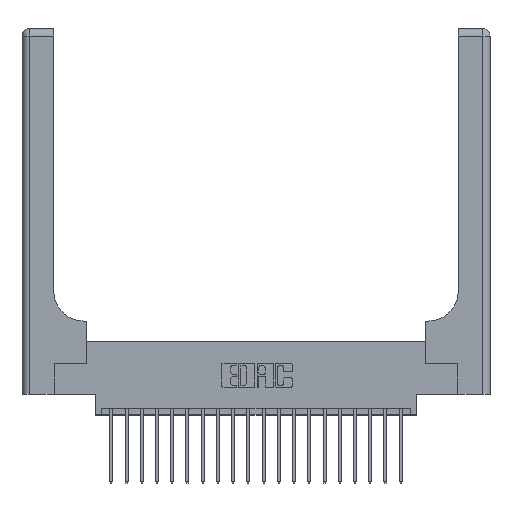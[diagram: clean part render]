
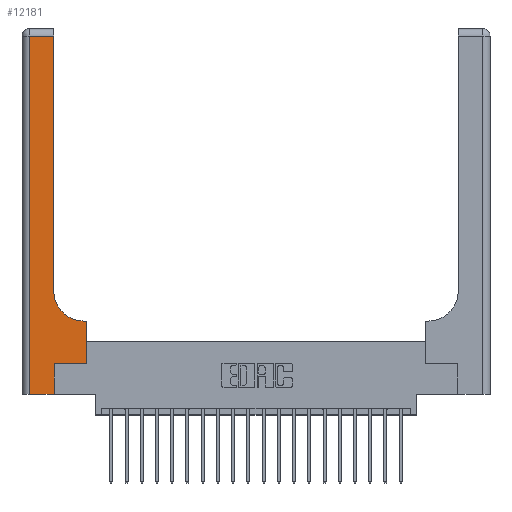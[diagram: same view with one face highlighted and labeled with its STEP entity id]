
A CAD part, top view. The second image highlights one B-rep face of the part: STEP entity #12181.
In plain terms, the highlighted planar face has unit normal (0, 0, 1).
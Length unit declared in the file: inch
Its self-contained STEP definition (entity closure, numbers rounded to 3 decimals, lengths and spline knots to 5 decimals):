
#41 = DIRECTION ( 'NONE',  ( 0., 0., -1. ) ) ;
#228 = EDGE_CURVE ( 'NONE', #10021, #4223, #10165, .T. ) ;
#244 = CARTESIAN_POINT ( 'NONE',  ( 0.51, 0.85, 0.37 ) ) ;
#1099 = LINE ( 'NONE', #19202, #9352 ) ;
#1638 = EDGE_CURVE ( 'NONE', #3198, #4495, #20206, .T. ) ;
#1724 = LINE ( 'NONE', #20280, #9957 ) ;
#1921 = DIRECTION ( 'NONE',  ( 1., 0., 0. ) ) ;
#1923 = EDGE_CURVE ( 'NONE', #4495, #19220, #19425, .T. ) ;
#2219 = EDGE_CURVE ( 'NONE', #4223, #13548, #1099, .T. ) ;
#2517 = DIRECTION ( 'NONE',  ( -1., 0., 0. ) ) ;
#2834 = EDGE_CURVE ( 'NONE', #20882, #5287, #16561, .T. ) ;
#2961 = ORIENTED_EDGE ( 'NONE', *, *, #7154, .T. ) ;
#3005 = CARTESIAN_POINT ( 'NONE',  ( 0.26, 0.85, 0.37 ) ) ;
#3198 = VERTEX_POINT ( 'NONE', #14368 ) ;
#3259 = CARTESIAN_POINT ( 'NONE',  ( 0.528, 0.25, 0.37 ) ) ;
#3377 = VECTOR ( 'NONE', #16233, 39.37008 ) ;
#4223 = VERTEX_POINT ( 'NONE', #15174 ) ;
#4400 = ORIENTED_EDGE ( 'NONE', *, *, #19896, .T. ) ;
#4495 = VERTEX_POINT ( 'NONE', #6256 ) ;
#4702 = CARTESIAN_POINT ( 'NONE',  ( 0.06, 2.94, 0.37 ) ) ;
#5287 = VERTEX_POINT ( 'NONE', #4702 ) ;
#5304 = ORIENTED_EDGE ( 'NONE', *, *, #1638, .T. ) ;
#5345 = CARTESIAN_POINT ( 'NONE',  ( 0.06, 3., 0.37 ) ) ;
#6256 = CARTESIAN_POINT ( 'NONE',  ( 0.51, 0.6, 0.37 ) ) ;
#6871 = ORIENTED_EDGE ( 'NONE', *, *, #13580, .T. ) ;
#6963 = CARTESIAN_POINT ( 'NONE',  ( 0.265, 0., 0.37 ) ) ;
#7154 = EDGE_CURVE ( 'NONE', #13548, #3198, #20515, .T. ) ;
#7788 = VECTOR ( 'NONE', #19711, 39.37008 ) ;
#8278 = CARTESIAN_POINT ( 'NONE',  ( 0., 3., 0.37 ) ) ;
#8467 = EDGE_LOOP ( 'NONE', ( #4400, #9525, #6871, #11680, #15297, #10908, #2961, #5304, #20323 ) ) ;
#9001 = CARTESIAN_POINT ( 'NONE',  ( 0.265, 0., 0.37 ) ) ;
#9352 = VECTOR ( 'NONE', #17563, 39.37008 ) ;
#9525 = ORIENTED_EDGE ( 'NONE', *, *, #2834, .T. ) ;
#9832 = CARTESIAN_POINT ( 'NONE',  ( 0., 2.94, 0.37 ) ) ;
#9928 = PLANE ( 'NONE',  #16581 ) ;
#9957 = VECTOR ( 'NONE', #18627, 39.37008 ) ;
#10021 = VERTEX_POINT ( 'NONE', #9001 ) ;
#10165 = LINE ( 'NONE', #6963, #14561 ) ;
#10302 = VECTOR ( 'NONE', #18523, 39.37008 ) ;
#10415 = CARTESIAN_POINT ( 'NONE',  ( 0.26, 2.94, 0.37 ) ) ;
#10723 = CARTESIAN_POINT ( 'NONE',  ( 0.26, 0.6, 0.37 ) ) ;
#10908 = ORIENTED_EDGE ( 'NONE', *, *, #2219, .T. ) ;
#11462 = VECTOR ( 'NONE', #2517, 39.37008 ) ;
#11603 = DIRECTION ( 'NONE',  ( -1., 0., 0. ) ) ;
#11680 = ORIENTED_EDGE ( 'NONE', *, *, #15737, .T. ) ;
#11787 = DIRECTION ( 'NONE',  ( 0., 0., -1. ) ) ;
#12139 = LINE ( 'NONE', #21199, #3377 ) ;
#12181 = ADVANCED_FACE ( 'NONE', ( #16476 ), #9928, .F. ) ;
#12770 = VECTOR ( 'NONE', #14773, 39.37008 ) ;
#13548 = VERTEX_POINT ( 'NONE', #18453 ) ;
#13580 = EDGE_CURVE ( 'NONE', #5287, #19436, #19087, .T. ) ;
#14368 = CARTESIAN_POINT ( 'NONE',  ( 0.528, 0.6, 0.37 ) ) ;
#14561 = VECTOR ( 'NONE', #18494, 39.37008 ) ;
#14773 = DIRECTION ( 'NONE',  ( 0., 1., 0. ) ) ;
#15174 = CARTESIAN_POINT ( 'NONE',  ( 0.265, 0.25, 0.37 ) ) ;
#15297 = ORIENTED_EDGE ( 'NONE', *, *, #228, .T. ) ;
#15737 = EDGE_CURVE ( 'NONE', #19436, #10021, #1724, .T. ) ;
#16233 = DIRECTION ( 'NONE',  ( 0., 1., 0. ) ) ;
#16476 = FACE_OUTER_BOUND ( 'NONE', #8467, .T. ) ;
#16561 = LINE ( 'NONE', #9832, #7788 ) ;
#16581 = AXIS2_PLACEMENT_3D ( 'NONE', #8278, #41, #11603 ) ;
#16689 = CARTESIAN_POINT ( 'NONE',  ( 0.06, 0., 0.37 ) ) ;
#17563 = DIRECTION ( 'NONE',  ( 1., 0., 0. ) ) ;
#18453 = CARTESIAN_POINT ( 'NONE',  ( 0.528, 0.25, 0.37 ) ) ;
#18494 = DIRECTION ( 'NONE',  ( 0., 1., 0. ) ) ;
#18523 = DIRECTION ( 'NONE',  ( 0., -1., 0. ) ) ;
#18627 = DIRECTION ( 'NONE',  ( 1., 0., 0. ) ) ;
#19087 = LINE ( 'NONE', #5345, #10302 ) ;
#19202 = CARTESIAN_POINT ( 'NONE',  ( 0.265, 0.25, 0.37 ) ) ;
#19220 = VERTEX_POINT ( 'NONE', #3005 ) ;
#19425 = CIRCLE ( 'NONE', #20367, 0.25 ) ;
#19436 = VERTEX_POINT ( 'NONE', #16689 ) ;
#19711 = DIRECTION ( 'NONE',  ( -1., 0., 0. ) ) ;
#19896 = EDGE_CURVE ( 'NONE', #19220, #20882, #12139, .T. ) ;
#20206 = LINE ( 'NONE', #10723, #11462 ) ;
#20280 = CARTESIAN_POINT ( 'NONE',  ( 0., 0., 0.37 ) ) ;
#20323 = ORIENTED_EDGE ( 'NONE', *, *, #1923, .T. ) ;
#20367 = AXIS2_PLACEMENT_3D ( 'NONE', #244, #11787, #1921 ) ;
#20515 = LINE ( 'NONE', #3259, #12770 ) ;
#20882 = VERTEX_POINT ( 'NONE', #10415 ) ;
#21199 = CARTESIAN_POINT ( 'NONE',  ( 0.26, 3., 0.37 ) ) ;
